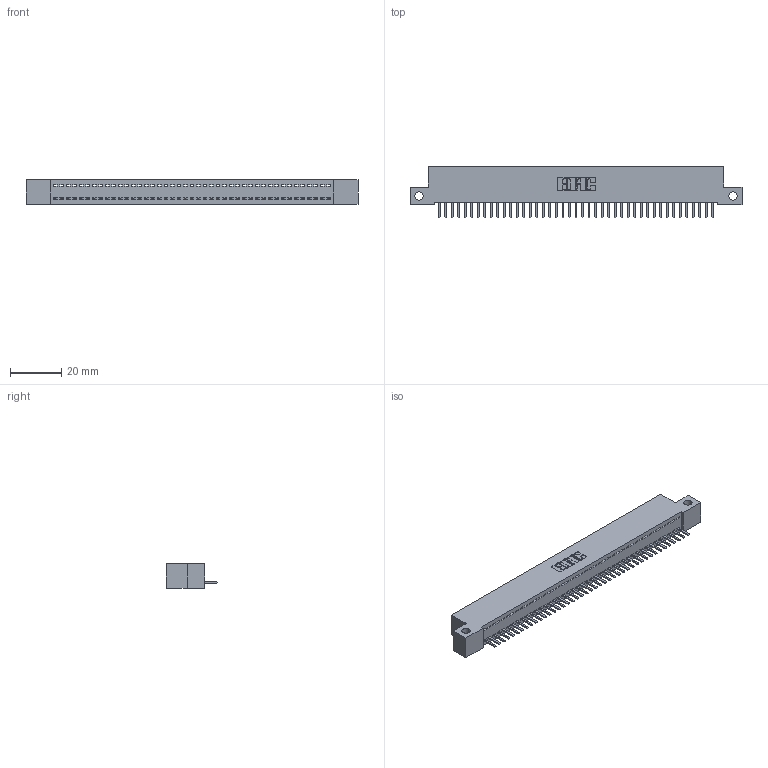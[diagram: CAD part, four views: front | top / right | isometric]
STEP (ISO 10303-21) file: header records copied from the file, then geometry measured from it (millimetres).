
FILE_DESCRIPTION (( 'STEP AP203' ), '1' );
FILE_NAME ('392-043-520-112.STEP', '2018-08-16T14:13:33', ( '' ), ( '' ), 'SwSTEP 2.0', 'SolidWorks 2016', '' );
FILE_SCHEMA (( 'CONFIG_CONTROL_DESIGN' ));
Length unit declared in the file: inch
Products named in the file (3): 342 Part_Side Mount; 345-292-001_345-293-120; 392-043-520-112
Assembly tree (44 placements, depth 2):
  392-043-520-112
    342 Part_Side Mount
    345-292-001_345-293-120  x43
Bounding box: 129.54 x 20.02 x 9.4 mm (x, y, z)
Volume: 11164.1 mm3; surface area: 15854 mm2
Topology: 44 solids, 44 shells, 2776 faces, 8211 edges, 5358 vertices
Faces by surface type: plane 1958, cylinder 818
Entity records: 26143 total; most frequent: CARTESIAN_POINT 4527, ORIENTED_EDGE 4494, DIRECTION 3805, EDGE_CURVE 2247, LINE 2115, VECTOR 2115, VERTEX_POINT 1494, AXIS2_PLACEMENT_3D 845
